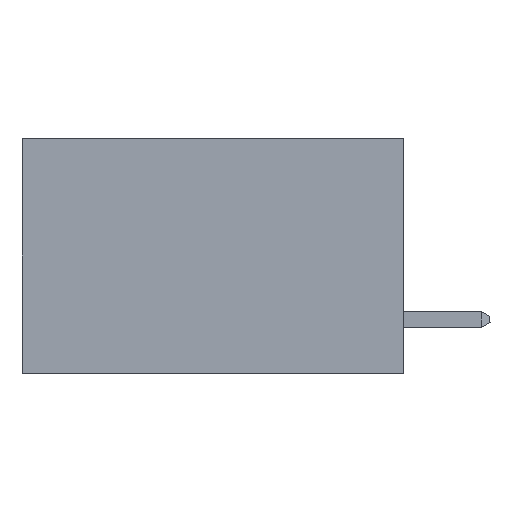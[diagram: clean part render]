
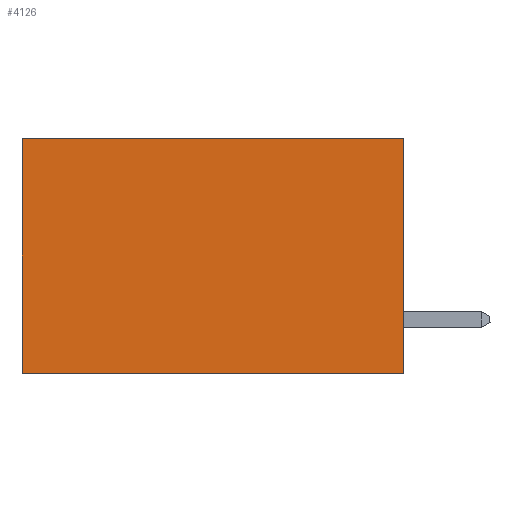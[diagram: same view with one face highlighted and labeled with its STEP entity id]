
A CAD part, left-side view. The second image highlights one B-rep face of the part: STEP entity #4126.
In plain terms, the highlighted planar face has unit normal (-1, 0, 0).
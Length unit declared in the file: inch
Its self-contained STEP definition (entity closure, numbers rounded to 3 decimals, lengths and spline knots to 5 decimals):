
#677 = CARTESIAN_POINT ( 'NONE',  ( 0.2875, 0., -0.37 ) ) ;
#1870 = EDGE_LOOP ( 'NONE', ( #10411, #24539, #22444, #16088 ) ) ;
#1896 = FACE_OUTER_BOUND ( 'NONE', #1870, .T. ) ;
#3882 = EDGE_CURVE ( 'NONE', #14914, #17441, #12578, .T. ) ;
#4126 = ADVANCED_FACE ( 'NONE', ( #1896 ), #4901, .F. ) ;
#4480 = CARTESIAN_POINT ( 'NONE',  ( 0.2875, 0., 0. ) ) ;
#4901 = PLANE ( 'NONE',  #7184 ) ;
#5251 = CARTESIAN_POINT ( 'NONE',  ( 0.2875, 0.6, 0. ) ) ;
#6916 = DIRECTION ( 'NONE',  ( 0., 0., -1. ) ) ;
#7184 = AXIS2_PLACEMENT_3D ( 'NONE', #16597, #18513, #6916 ) ;
#7410 = DIRECTION ( 'NONE',  ( 0., 0., -1. ) ) ;
#9179 = VECTOR ( 'NONE', #21960, 39.37008 ) ;
#9310 = VERTEX_POINT ( 'NONE', #14604 ) ;
#10037 = CARTESIAN_POINT ( 'NONE',  ( 0.2875, 0., 0. ) ) ;
#10147 = LINE ( 'NONE', #5251, #24912 ) ;
#10411 = ORIENTED_EDGE ( 'NONE', *, *, #14594, .T. ) ;
#11957 = DIRECTION ( 'NONE',  ( 0., 0., -1. ) ) ;
#12578 = LINE ( 'NONE', #10037, #17821 ) ;
#13953 = VERTEX_POINT ( 'NONE', #23515 ) ;
#14084 = CARTESIAN_POINT ( 'NONE',  ( 0.2875, 0., -0.37 ) ) ;
#14338 = LINE ( 'NONE', #4480, #9179 ) ;
#14594 = EDGE_CURVE ( 'NONE', #13953, #9310, #10147, .T. ) ;
#14604 = CARTESIAN_POINT ( 'NONE',  ( 0.2875, 0.6, -0.37 ) ) ;
#14914 = VERTEX_POINT ( 'NONE', #20359 ) ;
#16088 = ORIENTED_EDGE ( 'NONE', *, *, #16150, .T. ) ;
#16150 = EDGE_CURVE ( 'NONE', #14914, #13953, #14338, .T. ) ;
#16597 = CARTESIAN_POINT ( 'NONE',  ( 0.2875, 0., 0. ) ) ;
#17441 = VERTEX_POINT ( 'NONE', #677 ) ;
#17821 = VECTOR ( 'NONE', #11957, 39.37008 ) ;
#18513 = DIRECTION ( 'NONE',  ( 1., 0., 0. ) ) ;
#19337 = LINE ( 'NONE', #14084, #21746 ) ;
#20359 = CARTESIAN_POINT ( 'NONE',  ( 0.2875, 0., 0. ) ) ;
#21746 = VECTOR ( 'NONE', #21757, 39.37008 ) ;
#21757 = DIRECTION ( 'NONE',  ( 0., 1., 0. ) ) ;
#21960 = DIRECTION ( 'NONE',  ( 0., 1., 0. ) ) ;
#22444 = ORIENTED_EDGE ( 'NONE', *, *, #3882, .F. ) ;
#23515 = CARTESIAN_POINT ( 'NONE',  ( 0.2875, 0.6, 0. ) ) ;
#24145 = EDGE_CURVE ( 'NONE', #17441, #9310, #19337, .T. ) ;
#24539 = ORIENTED_EDGE ( 'NONE', *, *, #24145, .F. ) ;
#24912 = VECTOR ( 'NONE', #7410, 39.37008 ) ;
